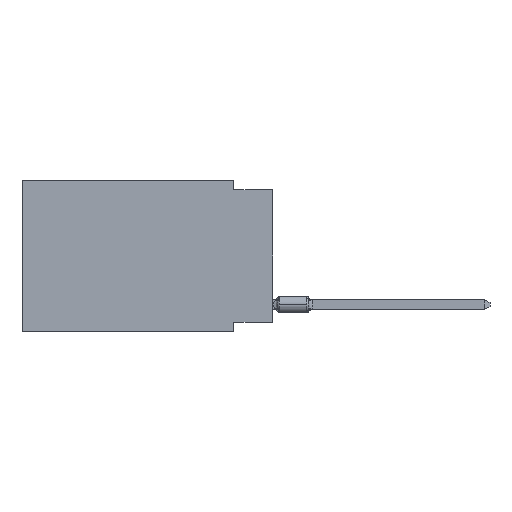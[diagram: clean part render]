
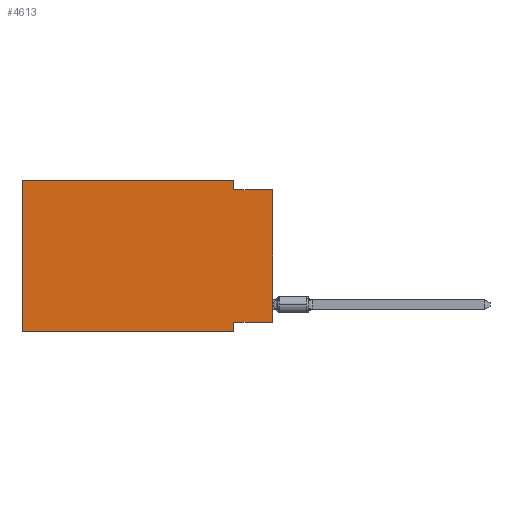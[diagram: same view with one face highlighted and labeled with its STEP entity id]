
A CAD part, left-side view. The second image highlights one B-rep face of the part: STEP entity #4613.
In plain terms, the highlighted planar face has unit normal (-1, 0, 0).
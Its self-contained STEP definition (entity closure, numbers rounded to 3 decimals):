
#232 = VERTEX_POINT ( 'NONE', #2281 ) ;
#356 = DIRECTION ( 'NONE',  ( 0., 0., -1. ) ) ;
#388 = PLANE ( 'NONE',  #1245 ) ;
#629 = DIRECTION ( 'NONE',  ( 0., -1., 0. ) ) ;
#774 = LINE ( 'NONE', #12891, #6384 ) ;
#1245 = AXIS2_PLACEMENT_3D ( 'NONE', #16128, #9012, #9455 ) ;
#1535 = ORIENTED_EDGE ( 'NONE', *, *, #9135, .F. ) ;
#1571 = VERTEX_POINT ( 'NONE', #6732 ) ;
#1686 = LINE ( 'NONE', #3701, #14884 ) ;
#2281 = CARTESIAN_POINT ( 'NONE',  ( 0., 16.383, 0. ) ) ;
#2284 = VECTOR ( 'NONE', #16576, 1000. ) ;
#2345 = CARTESIAN_POINT ( 'NONE',  ( 0., 2.54, -0.635 ) ) ;
#2539 = EDGE_CURVE ( 'NONE', #5909, #3909, #10183, .T. ) ;
#2568 = EDGE_CURVE ( 'NONE', #9669, #3909, #1686, .T. ) ;
#2779 = CARTESIAN_POINT ( 'NONE',  ( 0., 2.54, -9.271 ) ) ;
#3015 = VECTOR ( 'NONE', #629, 1000. ) ;
#3038 = CARTESIAN_POINT ( 'NONE',  ( 0., 0., -0.635 ) ) ;
#3525 = EDGE_LOOP ( 'NONE', ( #13752, #15373, #1535, #9632, #4551, #6311, #3680, #11358 ) ) ;
#3632 = CARTESIAN_POINT ( 'NONE',  ( 0., 2.54, -9.906 ) ) ;
#3680 = ORIENTED_EDGE ( 'NONE', *, *, #4916, .F. ) ;
#3701 = CARTESIAN_POINT ( 'NONE',  ( 0., 0., 0. ) ) ;
#3909 = VERTEX_POINT ( 'NONE', #12283 ) ;
#4006 = CARTESIAN_POINT ( 'NONE',  ( 0., 16.383, -9.906 ) ) ;
#4240 = CARTESIAN_POINT ( 'NONE',  ( 0., 16.383, 0. ) ) ;
#4551 = ORIENTED_EDGE ( 'NONE', *, *, #6281, .F. ) ;
#4613 = ADVANCED_FACE ( 'NONE', ( #5946 ), #388, .F. ) ;
#4916 = EDGE_CURVE ( 'NONE', #12870, #6418, #14046, .T. ) ;
#5403 = DIRECTION ( 'NONE',  ( 0., 0., 1. ) ) ;
#5838 = LINE ( 'NONE', #4006, #3015 ) ;
#5909 = VERTEX_POINT ( 'NONE', #2345 ) ;
#5946 = FACE_OUTER_BOUND ( 'NONE', #3525, .T. ) ;
#6281 = EDGE_CURVE ( 'NONE', #15423, #232, #774, .T. ) ;
#6311 = ORIENTED_EDGE ( 'NONE', *, *, #18437, .T. ) ;
#6384 = VECTOR ( 'NONE', #11295, 1000. ) ;
#6418 = VERTEX_POINT ( 'NONE', #16010 ) ;
#6732 = CARTESIAN_POINT ( 'NONE',  ( 0., 2.54, 0. ) ) ;
#8732 = CARTESIAN_POINT ( 'NONE',  ( 0., 0., -9.271 ) ) ;
#9012 = DIRECTION ( 'NONE',  ( 1., 0., 0. ) ) ;
#9135 = EDGE_CURVE ( 'NONE', #1571, #5909, #21668, .T. ) ;
#9455 = DIRECTION ( 'NONE',  ( 0., 0., -1. ) ) ;
#9632 = ORIENTED_EDGE ( 'NONE', *, *, #17695, .F. ) ;
#9669 = VERTEX_POINT ( 'NONE', #8732 ) ;
#10183 = LINE ( 'NONE', #3038, #17401 ) ;
#10335 = CARTESIAN_POINT ( 'NONE',  ( 0., 16.383, -9.906 ) ) ;
#10579 = CARTESIAN_POINT ( 'NONE',  ( 0., 0., -9.271 ) ) ;
#10664 = VECTOR ( 'NONE', #356, 1000. ) ;
#11258 = LINE ( 'NONE', #4240, #2284 ) ;
#11295 = DIRECTION ( 'NONE',  ( 0., 0., 1. ) ) ;
#11358 = ORIENTED_EDGE ( 'NONE', *, *, #13000, .F. ) ;
#12055 = DIRECTION ( 'NONE',  ( 0., 1., 0. ) ) ;
#12283 = CARTESIAN_POINT ( 'NONE',  ( 0., 0., -0.635 ) ) ;
#12870 = VERTEX_POINT ( 'NONE', #2779 ) ;
#12891 = CARTESIAN_POINT ( 'NONE',  ( 0., 16.383, 0. ) ) ;
#12894 = VECTOR ( 'NONE', #12055, 1000. ) ;
#13000 = EDGE_CURVE ( 'NONE', #9669, #12870, #19165, .T. ) ;
#13752 = ORIENTED_EDGE ( 'NONE', *, *, #2568, .T. ) ;
#14046 = LINE ( 'NONE', #3632, #10664 ) ;
#14884 = VECTOR ( 'NONE', #5403, 1000. ) ;
#15373 = ORIENTED_EDGE ( 'NONE', *, *, #2539, .F. ) ;
#15423 = VERTEX_POINT ( 'NONE', #10335 ) ;
#16010 = CARTESIAN_POINT ( 'NONE',  ( 0., 2.54, -9.906 ) ) ;
#16128 = CARTESIAN_POINT ( 'NONE',  ( 0., 16.383, 0. ) ) ;
#16576 = DIRECTION ( 'NONE',  ( 0., -1., 0. ) ) ;
#17401 = VECTOR ( 'NONE', #22060, 1000. ) ;
#17695 = EDGE_CURVE ( 'NONE', #232, #1571, #11258, .T. ) ;
#18370 = CARTESIAN_POINT ( 'NONE',  ( 0., 2.54, 0. ) ) ;
#18437 = EDGE_CURVE ( 'NONE', #15423, #6418, #5838, .T. ) ;
#19165 = LINE ( 'NONE', #10579, #12894 ) ;
#20077 = DIRECTION ( 'NONE',  ( 0., 0., -1. ) ) ;
#21668 = LINE ( 'NONE', #18370, #22211 ) ;
#22060 = DIRECTION ( 'NONE',  ( 0., -1., 0. ) ) ;
#22211 = VECTOR ( 'NONE', #20077, 1000. ) ;
